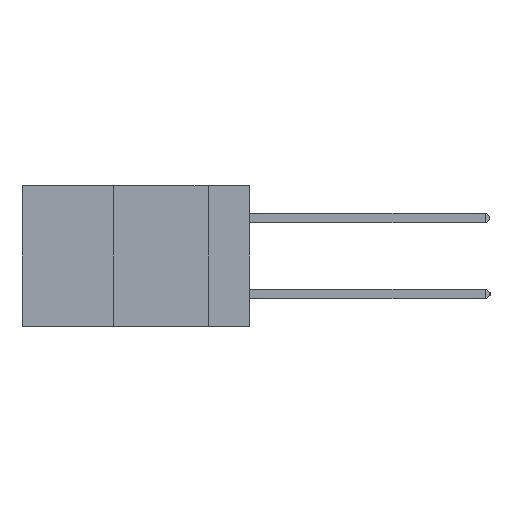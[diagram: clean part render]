
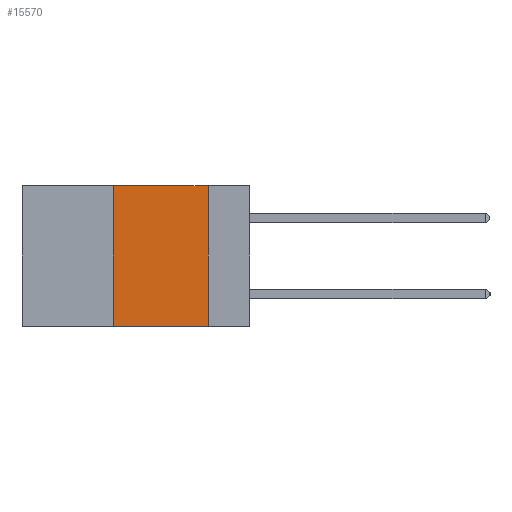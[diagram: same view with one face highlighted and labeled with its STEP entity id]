
A CAD part, left-side view. The second image highlights one B-rep face of the part: STEP entity #15570.
In plain terms, the highlighted planar face has unit normal (-1, 0, 0).
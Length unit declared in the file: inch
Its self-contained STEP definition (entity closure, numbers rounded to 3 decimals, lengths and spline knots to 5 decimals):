
#404 = EDGE_CURVE ( 'NONE', #15391, #19073, #7989, .T. ) ;
#658 = LINE ( 'NONE', #2359, #5335 ) ;
#1093 = CARTESIAN_POINT ( 'NONE',  ( 0., 0.11, -0.37 ) ) ;
#1815 = FACE_OUTER_BOUND ( 'NONE', #19716, .T. ) ;
#2071 = CARTESIAN_POINT ( 'NONE',  ( 0., 0.6, 0. ) ) ;
#2300 = VERTEX_POINT ( 'NONE', #1093 ) ;
#2359 = CARTESIAN_POINT ( 'NONE',  ( 0., 0.11, 0. ) ) ;
#3264 = VECTOR ( 'NONE', #3514, 39.37008 ) ;
#3369 = CARTESIAN_POINT ( 'NONE',  ( 0., 0.6, -0.37 ) ) ;
#3514 = DIRECTION ( 'NONE',  ( 0., -1., 0. ) ) ;
#3830 = PLANE ( 'NONE',  #4749 ) ;
#4749 = AXIS2_PLACEMENT_3D ( 'NONE', #2071, #17839, #7395 ) ;
#5320 = EDGE_CURVE ( 'NONE', #16135, #2300, #7409, .T. ) ;
#5335 = VECTOR ( 'NONE', #21508, 39.37008 ) ;
#5770 = CARTESIAN_POINT ( 'NONE',  ( 0., 0.36, 0. ) ) ;
#7254 = ORIENTED_EDGE ( 'NONE', *, *, #13685, .F. ) ;
#7395 = DIRECTION ( 'NONE',  ( 0., 0., -1. ) ) ;
#7409 = LINE ( 'NONE', #3369, #3264 ) ;
#7989 = LINE ( 'NONE', #12931, #12101 ) ;
#9385 = LINE ( 'NONE', #5770, #13513 ) ;
#10261 = ORIENTED_EDGE ( 'NONE', *, *, #11896, .F. ) ;
#10665 = CARTESIAN_POINT ( 'NONE',  ( 0., 0.36, -0.37 ) ) ;
#11105 = ORIENTED_EDGE ( 'NONE', *, *, #5320, .T. ) ;
#11896 = EDGE_CURVE ( 'NONE', #19073, #2300, #658, .T. ) ;
#12101 = VECTOR ( 'NONE', #16713, 39.37008 ) ;
#12733 = DIRECTION ( 'NONE',  ( 0., 0., 1. ) ) ;
#12931 = CARTESIAN_POINT ( 'NONE',  ( 0., 0.6, 0. ) ) ;
#13513 = VECTOR ( 'NONE', #12733, 39.37008 ) ;
#13685 = EDGE_CURVE ( 'NONE', #16135, #15391, #9385, .T. ) ;
#14460 = CARTESIAN_POINT ( 'NONE',  ( 0., 0.11, 0. ) ) ;
#15391 = VERTEX_POINT ( 'NONE', #19062 ) ;
#15570 = ADVANCED_FACE ( 'NONE', ( #1815 ), #3830, .F. ) ;
#16135 = VERTEX_POINT ( 'NONE', #10665 ) ;
#16713 = DIRECTION ( 'NONE',  ( 0., -1., 0. ) ) ;
#17839 = DIRECTION ( 'NONE',  ( 1., 0., 0. ) ) ;
#19062 = CARTESIAN_POINT ( 'NONE',  ( 0., 0.36, 0. ) ) ;
#19073 = VERTEX_POINT ( 'NONE', #14460 ) ;
#19520 = ORIENTED_EDGE ( 'NONE', *, *, #404, .F. ) ;
#19716 = EDGE_LOOP ( 'NONE', ( #10261, #19520, #7254, #11105 ) ) ;
#21508 = DIRECTION ( 'NONE',  ( 0., 0., -1. ) ) ;
